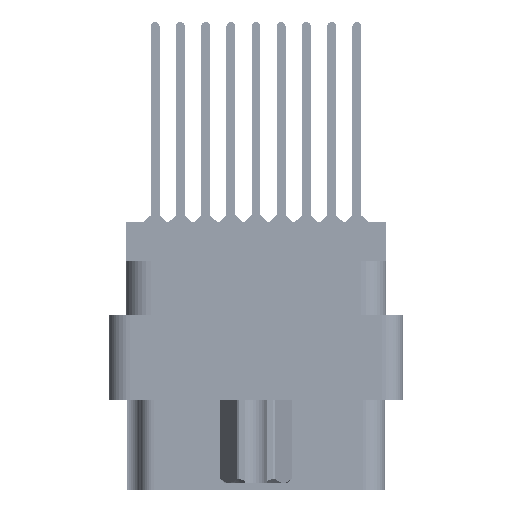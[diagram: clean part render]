
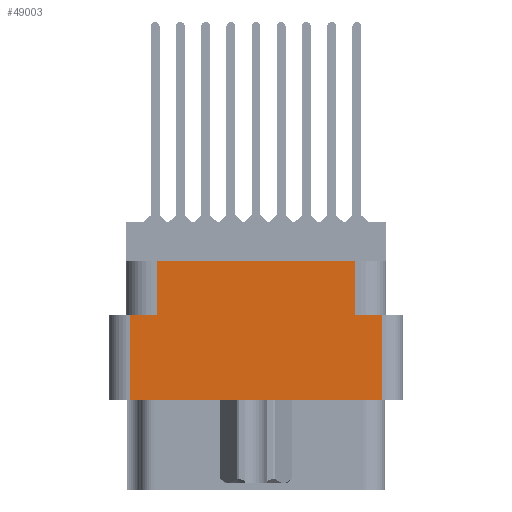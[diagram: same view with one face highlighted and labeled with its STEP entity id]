
A CAD part, left-side view. The second image highlights one B-rep face of the part: STEP entity #49003.
In plain terms, the highlighted planar face has unit normal (-1, 0, 0).
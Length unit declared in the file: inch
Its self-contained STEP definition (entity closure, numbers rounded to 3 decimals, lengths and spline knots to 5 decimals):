
#70 = DIRECTION ( 'NONE',  ( 0., 0., 1. ) ) ;
#141 = EDGE_LOOP ( 'NONE', ( #1424, #56168, #19460, #5755, #51015, #18590, #9565, #14736 ) ) ;
#274 = VERTEX_POINT ( 'NONE', #33386 ) ;
#1424 = ORIENTED_EDGE ( 'NONE', *, *, #57980, .F. ) ;
#5755 = ORIENTED_EDGE ( 'NONE', *, *, #15712, .T. ) ;
#6813 = CARTESIAN_POINT ( 'NONE',  ( -1.296, -0.296, -0.277 ) ) ;
#6838 = VECTOR ( 'NONE', #53354, 39.37008 ) ;
#7879 = VECTOR ( 'NONE', #43930, 39.37008 ) ;
#8224 = EDGE_CURVE ( 'NONE', #42162, #274, #42359, .T. ) ;
#8528 = DIRECTION ( 'NONE',  ( -1., 0., 0. ) ) ;
#9121 = DIRECTION ( 'NONE',  ( 0., 0., 1. ) ) ;
#9565 = ORIENTED_EDGE ( 'NONE', *, *, #55859, .F. ) ;
#10661 = EDGE_CURVE ( 'NONE', #10845, #14646, #33900, .T. ) ;
#10845 = VERTEX_POINT ( 'NONE', #24318 ) ;
#11373 = CARTESIAN_POINT ( 'NONE',  ( -1.296, 0.376, -0.798 ) ) ;
#14415 = VECTOR ( 'NONE', #48629, 39.37008 ) ;
#14646 = VERTEX_POINT ( 'NONE', #25336 ) ;
#14675 = LINE ( 'NONE', #31394, #28419 ) ;
#14736 = ORIENTED_EDGE ( 'NONE', *, *, #8224, .F. ) ;
#15712 = EDGE_CURVE ( 'NONE', #43475, #51822, #37718, .T. ) ;
#18590 = ORIENTED_EDGE ( 'NONE', *, *, #50000, .T. ) ;
#18731 = CARTESIAN_POINT ( 'NONE',  ( -1.296, 0.438, -0.117 ) ) ;
#19349 = CARTESIAN_POINT ( 'NONE',  ( -1.296, 0., -0.529 ) ) ;
#19460 = ORIENTED_EDGE ( 'NONE', *, *, #25555, .F. ) ;
#19733 = CARTESIAN_POINT ( 'NONE',  ( -1.296, -0.376, -0.529 ) ) ;
#20902 = LINE ( 'NONE', #6813, #14415 ) ;
#21678 = DIRECTION ( 'NONE',  ( 0., -1., 0. ) ) ;
#24318 = CARTESIAN_POINT ( 'NONE',  ( -1.296, 0.376, -0.277 ) ) ;
#24979 = VECTOR ( 'NONE', #70, 39.37008 ) ;
#25336 = CARTESIAN_POINT ( 'NONE',  ( -1.296, 0.376, -0.529 ) ) ;
#25555 = EDGE_CURVE ( 'NONE', #43475, #14646, #53139, .T. ) ;
#26459 = CARTESIAN_POINT ( 'NONE',  ( -1.296, -0.376, -0.277 ) ) ;
#27837 = CARTESIAN_POINT ( 'NONE',  ( -1.296, -0.296, -0.117 ) ) ;
#28419 = VECTOR ( 'NONE', #21678, 39.37008 ) ;
#28680 = CARTESIAN_POINT ( 'NONE',  ( -1.296, -0.376, -0.798 ) ) ;
#31394 = CARTESIAN_POINT ( 'NONE',  ( -1.296, 0., -0.277 ) ) ;
#32311 = LINE ( 'NONE', #18731, #43163 ) ;
#33386 = CARTESIAN_POINT ( 'NONE',  ( -1.296, 0.296, -0.117 ) ) ;
#33464 = VERTEX_POINT ( 'NONE', #27837 ) ;
#33900 = LINE ( 'NONE', #11373, #7879 ) ;
#35231 = PLANE ( 'NONE',  #53662 ) ;
#36299 = CARTESIAN_POINT ( 'NONE',  ( -1.296, 0., -0.277 ) ) ;
#37718 = LINE ( 'NONE', #28680, #54395 ) ;
#37989 = DIRECTION ( 'NONE',  ( 0., 0., 1. ) ) ;
#42162 = VERTEX_POINT ( 'NONE', #56987 ) ;
#42359 = LINE ( 'NONE', #55641, #24979 ) ;
#42473 = EDGE_CURVE ( 'NONE', #49944, #51822, #43071, .T. ) ;
#43071 = LINE ( 'NONE', #36299, #44535 ) ;
#43163 = VECTOR ( 'NONE', #51140, 39.37008 ) ;
#43183 = CARTESIAN_POINT ( 'NONE',  ( -1.296, -0.296, -0.277 ) ) ;
#43475 = VERTEX_POINT ( 'NONE', #19733 ) ;
#43930 = DIRECTION ( 'NONE',  ( 0., 0., -1. ) ) ;
#44535 = VECTOR ( 'NONE', #49419, 39.37008 ) ;
#48629 = DIRECTION ( 'NONE',  ( 0., 0., 1. ) ) ;
#49003 = ADVANCED_FACE ( 'NONE', ( #52925 ), #35231, .T. ) ;
#49168 = CARTESIAN_POINT ( 'NONE',  ( -1.296, -0.438, -0.798 ) ) ;
#49419 = DIRECTION ( 'NONE',  ( 0., -1., 0. ) ) ;
#49944 = VERTEX_POINT ( 'NONE', #43183 ) ;
#50000 = EDGE_CURVE ( 'NONE', #49944, #33464, #20902, .T. ) ;
#51015 = ORIENTED_EDGE ( 'NONE', *, *, #42473, .F. ) ;
#51140 = DIRECTION ( 'NONE',  ( 0., -1., 0. ) ) ;
#51822 = VERTEX_POINT ( 'NONE', #26459 ) ;
#52925 = FACE_OUTER_BOUND ( 'NONE', #141, .T. ) ;
#53139 = LINE ( 'NONE', #19349, #6838 ) ;
#53354 = DIRECTION ( 'NONE',  ( 0., 1., 0. ) ) ;
#53662 = AXIS2_PLACEMENT_3D ( 'NONE', #49168, #8528, #9121 ) ;
#54395 = VECTOR ( 'NONE', #37989, 39.37008 ) ;
#55641 = CARTESIAN_POINT ( 'NONE',  ( -1.296, 0.296, -0.277 ) ) ;
#55859 = EDGE_CURVE ( 'NONE', #274, #33464, #32311, .T. ) ;
#56168 = ORIENTED_EDGE ( 'NONE', *, *, #10661, .T. ) ;
#56987 = CARTESIAN_POINT ( 'NONE',  ( -1.296, 0.296, -0.277 ) ) ;
#57980 = EDGE_CURVE ( 'NONE', #10845, #42162, #14675, .T. ) ;
